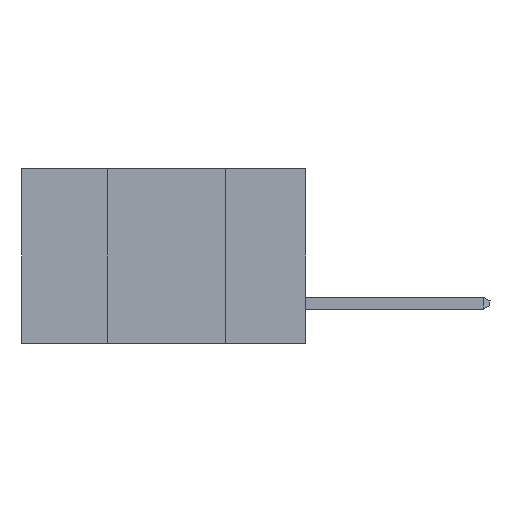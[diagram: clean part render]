
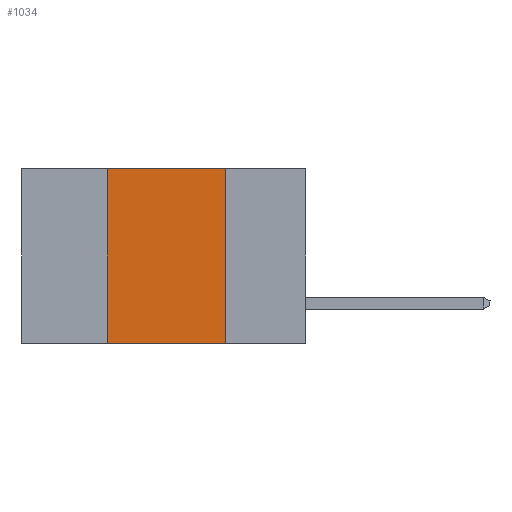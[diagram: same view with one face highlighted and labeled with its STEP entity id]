
A CAD part, left-side view. The second image highlights one B-rep face of the part: STEP entity #1034.
In plain terms, the highlighted planar face has unit normal (-1, 0, 0).
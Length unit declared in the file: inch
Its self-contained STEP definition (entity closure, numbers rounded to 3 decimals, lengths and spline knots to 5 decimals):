
#943 = ORIENTED_EDGE ( 'NONE', *, *, #8417, .F. ) ;
#1034 = ADVANCED_FACE ( 'NONE', ( #3684 ), #5218, .F. ) ;
#1859 = VECTOR ( 'NONE', #11184, 39.37008 ) ;
#2095 = EDGE_CURVE ( 'NONE', #16340, #15301, #16699, .T. ) ;
#2192 = ORIENTED_EDGE ( 'NONE', *, *, #16660, .T. ) ;
#2553 = DIRECTION ( 'NONE',  ( 0., -1., 0. ) ) ;
#2645 = CARTESIAN_POINT ( 'NONE',  ( 0., 0.6, -0.37 ) ) ;
#3497 = CARTESIAN_POINT ( 'NONE',  ( 0., 0.6, 0. ) ) ;
#3684 = FACE_OUTER_BOUND ( 'NONE', #12188, .T. ) ;
#4431 = VECTOR ( 'NONE', #6643, 39.37008 ) ;
#4450 = LINE ( 'NONE', #2645, #14205 ) ;
#5158 = AXIS2_PLACEMENT_3D ( 'NONE', #3497, #9518, #12202 ) ;
#5218 = PLANE ( 'NONE',  #5158 ) ;
#5338 = LINE ( 'NONE', #17170, #1859 ) ;
#5575 = EDGE_CURVE ( 'NONE', #15301, #7590, #14172, .T. ) ;
#6203 = DIRECTION ( 'NONE',  ( 0., 0., 1. ) ) ;
#6643 = DIRECTION ( 'NONE',  ( 0., -1., 0. ) ) ;
#7227 = CARTESIAN_POINT ( 'NONE',  ( 0., 0.17, 0. ) ) ;
#7366 = VERTEX_POINT ( 'NONE', #17897 ) ;
#7590 = VERTEX_POINT ( 'NONE', #7227 ) ;
#8417 = EDGE_CURVE ( 'NONE', #7590, #7366, #5338, .T. ) ;
#9142 = CARTESIAN_POINT ( 'NONE',  ( 0., 0.42, -0.37 ) ) ;
#9518 = DIRECTION ( 'NONE',  ( 1., 0., 0. ) ) ;
#9649 = VECTOR ( 'NONE', #6203, 39.37008 ) ;
#9733 = ORIENTED_EDGE ( 'NONE', *, *, #5575, .F. ) ;
#11184 = DIRECTION ( 'NONE',  ( 0., 0., -1. ) ) ;
#11592 = ORIENTED_EDGE ( 'NONE', *, *, #2095, .F. ) ;
#12188 = EDGE_LOOP ( 'NONE', ( #943, #9733, #11592, #2192 ) ) ;
#12202 = DIRECTION ( 'NONE',  ( 0., 0., -1. ) ) ;
#14172 = LINE ( 'NONE', #14263, #4431 ) ;
#14205 = VECTOR ( 'NONE', #2553, 39.37008 ) ;
#14263 = CARTESIAN_POINT ( 'NONE',  ( 0., 0.6, 0. ) ) ;
#14878 = CARTESIAN_POINT ( 'NONE',  ( 0., 0.42, -0.37 ) ) ;
#15301 = VERTEX_POINT ( 'NONE', #15530 ) ;
#15530 = CARTESIAN_POINT ( 'NONE',  ( 0., 0.42, 0. ) ) ;
#16340 = VERTEX_POINT ( 'NONE', #9142 ) ;
#16660 = EDGE_CURVE ( 'NONE', #16340, #7366, #4450, .T. ) ;
#16699 = LINE ( 'NONE', #14878, #9649 ) ;
#17170 = CARTESIAN_POINT ( 'NONE',  ( 0., 0.17, -0.37 ) ) ;
#17897 = CARTESIAN_POINT ( 'NONE',  ( 0., 0.17, -0.37 ) ) ;
